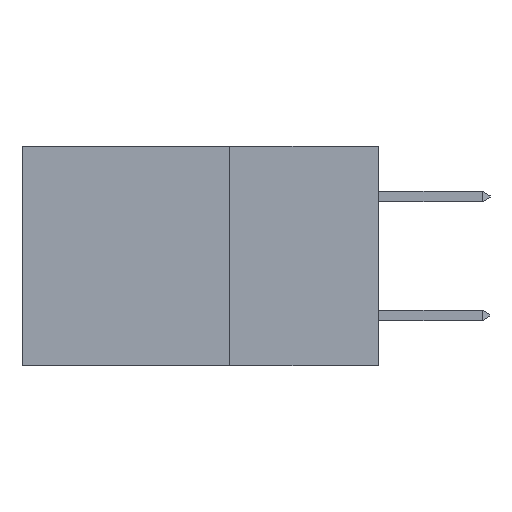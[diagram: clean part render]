
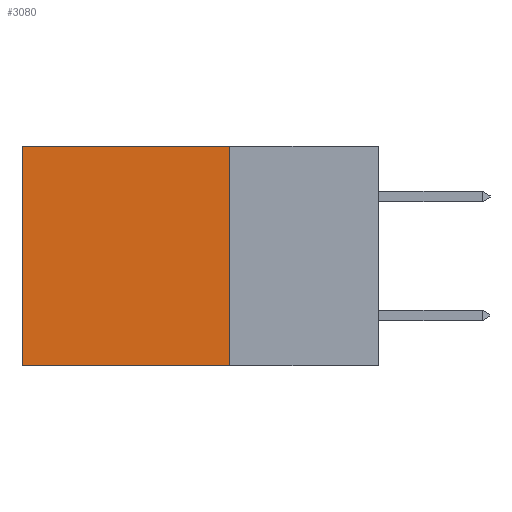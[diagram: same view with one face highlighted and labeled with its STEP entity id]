
A CAD part, left-side view. The second image highlights one B-rep face of the part: STEP entity #3080.
In plain terms, the highlighted planar face has unit normal (-1, 0, 0).
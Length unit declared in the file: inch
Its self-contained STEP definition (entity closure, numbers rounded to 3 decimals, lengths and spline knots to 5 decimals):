
#347 = CARTESIAN_POINT ( 'NONE',  ( 0.2615, 0.6, -0.37 ) ) ;
#357 = EDGE_CURVE ( 'NONE', #2829, #19445, #7495, .T. ) ;
#1820 = VECTOR ( 'NONE', #2909, 39.37008 ) ;
#2829 = VERTEX_POINT ( 'NONE', #8553 ) ;
#2909 = DIRECTION ( 'NONE',  ( 0., 1., 0. ) ) ;
#3080 = ADVANCED_FACE ( 'NONE', ( #11173 ), #3481, .F. ) ;
#3481 = PLANE ( 'NONE',  #19438 ) ;
#4594 = CARTESIAN_POINT ( 'NONE',  ( 0.2615, 0.25, -0.37 ) ) ;
#4608 = VECTOR ( 'NONE', #5494, 39.37008 ) ;
#5494 = DIRECTION ( 'NONE',  ( 0., 1., 0. ) ) ;
#5739 = DIRECTION ( 'NONE',  ( 0., 0., -1. ) ) ;
#6332 = VERTEX_POINT ( 'NONE', #16687 ) ;
#6909 = LINE ( 'NONE', #21482, #1820 ) ;
#7495 = LINE ( 'NONE', #347, #22237 ) ;
#8553 = CARTESIAN_POINT ( 'NONE',  ( 0.2615, 0.6, 0. ) ) ;
#8995 = EDGE_CURVE ( 'NONE', #6332, #2829, #14586, .T. ) ;
#9916 = ORIENTED_EDGE ( 'NONE', *, *, #8995, .T. ) ;
#10392 = EDGE_CURVE ( 'NONE', #6332, #14696, #19390, .T. ) ;
#10967 = CARTESIAN_POINT ( 'NONE',  ( 0.2615, 0.25, -0.37 ) ) ;
#11173 = FACE_OUTER_BOUND ( 'NONE', #12988, .T. ) ;
#12448 = ORIENTED_EDGE ( 'NONE', *, *, #10392, .F. ) ;
#12988 = EDGE_LOOP ( 'NONE', ( #18569, #23027, #12448, #9916 ) ) ;
#14586 = LINE ( 'NONE', #20362, #4608 ) ;
#14696 = VERTEX_POINT ( 'NONE', #17169 ) ;
#15782 = DIRECTION ( 'NONE',  ( 0., 0., -1. ) ) ;
#16687 = CARTESIAN_POINT ( 'NONE',  ( 0.2615, 0.25, 0. ) ) ;
#16891 = DIRECTION ( 'NONE',  ( 1., 0., 0. ) ) ;
#17169 = CARTESIAN_POINT ( 'NONE',  ( 0.2615, 0.25, -0.37 ) ) ;
#17640 = CARTESIAN_POINT ( 'NONE',  ( 0.2615, 0.6, -0.37 ) ) ;
#18238 = VECTOR ( 'NONE', #15782, 39.37008 ) ;
#18569 = ORIENTED_EDGE ( 'NONE', *, *, #357, .T. ) ;
#19390 = LINE ( 'NONE', #4594, #18238 ) ;
#19438 = AXIS2_PLACEMENT_3D ( 'NONE', #10967, #16891, #5739 ) ;
#19445 = VERTEX_POINT ( 'NONE', #17640 ) ;
#20039 = DIRECTION ( 'NONE',  ( 0., 0., -1. ) ) ;
#20202 = EDGE_CURVE ( 'NONE', #14696, #19445, #6909, .T. ) ;
#20362 = CARTESIAN_POINT ( 'NONE',  ( 0.2615, 0.25, 0. ) ) ;
#21482 = CARTESIAN_POINT ( 'NONE',  ( 0.2615, 0.25, -0.37 ) ) ;
#22237 = VECTOR ( 'NONE', #20039, 39.37008 ) ;
#23027 = ORIENTED_EDGE ( 'NONE', *, *, #20202, .F. ) ;
